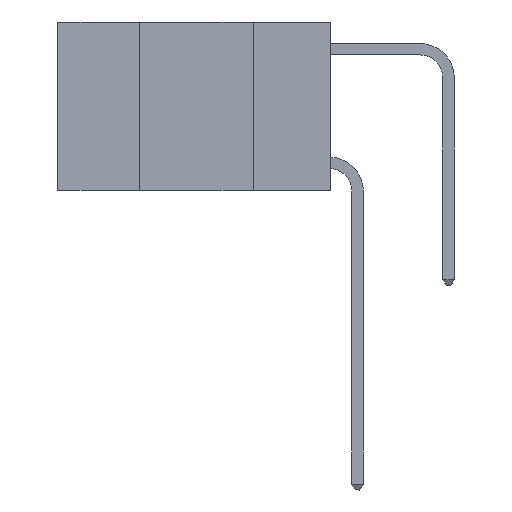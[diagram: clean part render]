
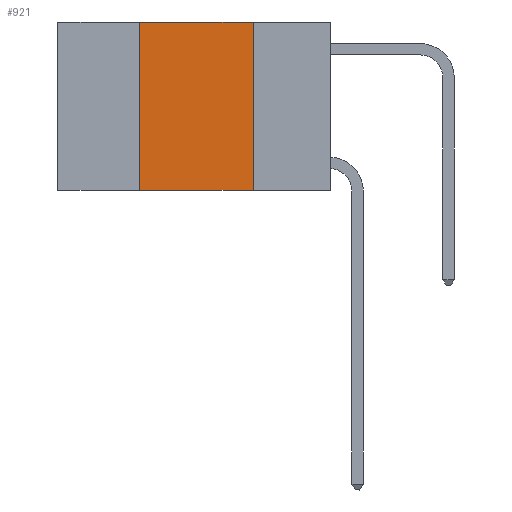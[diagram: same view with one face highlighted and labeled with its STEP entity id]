
A CAD part, left-side view. The second image highlights one B-rep face of the part: STEP entity #921.
In plain terms, the highlighted planar face has unit normal (-1, 0, 0).
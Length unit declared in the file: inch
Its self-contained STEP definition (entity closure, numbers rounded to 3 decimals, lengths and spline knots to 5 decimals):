
#347 = FACE_OUTER_BOUND ( 'NONE', #4337, .T. ) ;
#587 = LINE ( 'NONE', #5219, #5873 ) ;
#921 = ADVANCED_FACE ( 'NONE', ( #347 ), #7685, .F. ) ;
#1281 = CARTESIAN_POINT ( 'NONE',  ( 0., 0.42, 0. ) ) ;
#1534 = ORIENTED_EDGE ( 'NONE', *, *, #6483, .F. ) ;
#1546 = ORIENTED_EDGE ( 'NONE', *, *, #1799, .F. ) ;
#1690 = CARTESIAN_POINT ( 'NONE',  ( 0., 0.17, 0. ) ) ;
#1799 = EDGE_CURVE ( 'NONE', #11595, #3523, #587, .T. ) ;
#2995 = DIRECTION ( 'NONE',  ( 0., -1., 0. ) ) ;
#3523 = VERTEX_POINT ( 'NONE', #10007 ) ;
#3558 = LINE ( 'NONE', #1690, #8372 ) ;
#3790 = ORIENTED_EDGE ( 'NONE', *, *, #3999, .F. ) ;
#3946 = VECTOR ( 'NONE', #10692, 39.37008 ) ;
#3999 = EDGE_CURVE ( 'NONE', #10940, #11595, #7564, .T. ) ;
#4337 = EDGE_LOOP ( 'NONE', ( #1534, #1546, #3790, #8256 ) ) ;
#4632 = CARTESIAN_POINT ( 'NONE',  ( 0., 0.6, 0. ) ) ;
#5219 = CARTESIAN_POINT ( 'NONE',  ( 0., 0.6, 0. ) ) ;
#5873 = VECTOR ( 'NONE', #2995, 39.37008 ) ;
#6066 = VERTEX_POINT ( 'NONE', #12223 ) ;
#6380 = CARTESIAN_POINT ( 'NONE',  ( 0., 0.42, 0. ) ) ;
#6483 = EDGE_CURVE ( 'NONE', #3523, #6066, #3558, .T. ) ;
#7564 = LINE ( 'NONE', #1281, #9499 ) ;
#7685 = PLANE ( 'NONE',  #8556 ) ;
#8025 = DIRECTION ( 'NONE',  ( 0., 0., 1. ) ) ;
#8256 = ORIENTED_EDGE ( 'NONE', *, *, #10300, .T. ) ;
#8372 = VECTOR ( 'NONE', #8424, 39.37008 ) ;
#8424 = DIRECTION ( 'NONE',  ( 0., 0., -1. ) ) ;
#8475 = CARTESIAN_POINT ( 'NONE',  ( 0., 0.42, -0.37 ) ) ;
#8556 = AXIS2_PLACEMENT_3D ( 'NONE', #4632, #11333, #12345 ) ;
#8884 = LINE ( 'NONE', #10352, #3946 ) ;
#9499 = VECTOR ( 'NONE', #8025, 39.37008 ) ;
#10007 = CARTESIAN_POINT ( 'NONE',  ( 0., 0.17, 0. ) ) ;
#10300 = EDGE_CURVE ( 'NONE', #10940, #6066, #8884, .T. ) ;
#10352 = CARTESIAN_POINT ( 'NONE',  ( 0., 0.6, -0.37 ) ) ;
#10692 = DIRECTION ( 'NONE',  ( 0., -1., 0. ) ) ;
#10940 = VERTEX_POINT ( 'NONE', #8475 ) ;
#11333 = DIRECTION ( 'NONE',  ( 1., 0., 0. ) ) ;
#11595 = VERTEX_POINT ( 'NONE', #6380 ) ;
#12223 = CARTESIAN_POINT ( 'NONE',  ( 0., 0.17, -0.37 ) ) ;
#12345 = DIRECTION ( 'NONE',  ( 0., 0., -1. ) ) ;
